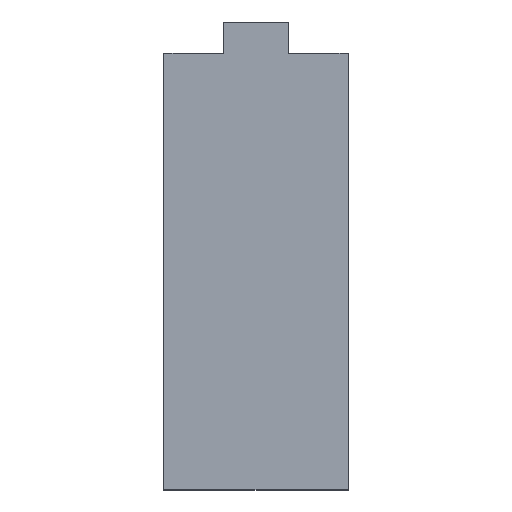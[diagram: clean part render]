
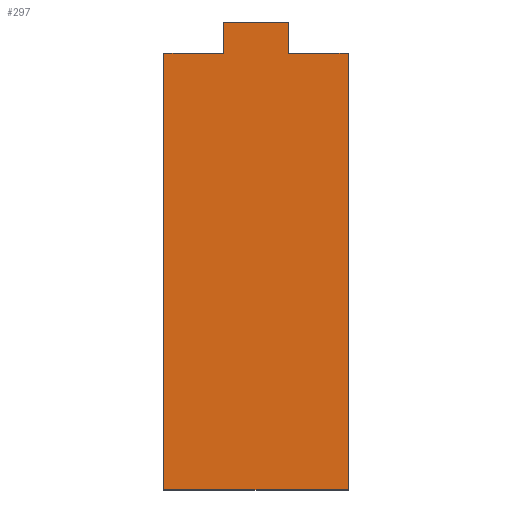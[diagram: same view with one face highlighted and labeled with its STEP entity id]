
A CAD part, top view. The second image highlights one B-rep face of the part: STEP entity #297.
In plain terms, the highlighted planar face has unit normal (0, 0, 1).
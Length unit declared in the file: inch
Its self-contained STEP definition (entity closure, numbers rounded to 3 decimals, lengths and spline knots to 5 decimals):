
#5 = DIRECTION ( 'NONE',  ( -1., 0., 0. ) ) ;
#11 = EDGE_CURVE ( 'NONE', #310, #309, #240, .T. ) ;
#15 = EDGE_CURVE ( 'NONE', #307, #330, #190, .T. ) ;
#16 = DIRECTION ( 'NONE',  ( 0., 1., 0. ) ) ;
#17 = CARTESIAN_POINT ( 'NONE',  ( 0.105, 1.4, 0.02 ) ) ;
#20 = CARTESIAN_POINT ( 'NONE',  ( 0., 0., 0.02 ) ) ;
#30 = CARTESIAN_POINT ( 'NONE',  ( -0.295, 1.4, 0.02 ) ) ;
#36 = PLANE ( 'NONE',  #134 ) ;
#39 = CARTESIAN_POINT ( 'NONE',  ( 0.295, 1.4, 0.02 ) ) ;
#58 = EDGE_CURVE ( 'NONE', #328, #325, #181, .T. ) ;
#60 = CARTESIAN_POINT ( 'NONE',  ( 0.295, 0., 0.02 ) ) ;
#61 = LINE ( 'NONE', #339, #225 ) ;
#72 = FACE_OUTER_BOUND ( 'NONE', #191, .T. ) ;
#79 = DIRECTION ( 'NONE',  ( 1., 0., 0. ) ) ;
#100 = CARTESIAN_POINT ( 'NONE',  ( 0.295, 0., 0.02 ) ) ;
#103 = EDGE_CURVE ( 'NONE', #322, #125, #168, .T. ) ;
#111 = VECTOR ( 'NONE', #228, 39.37008 ) ;
#118 = LINE ( 'NONE', #277, #111 ) ;
#125 = VERTEX_POINT ( 'NONE', #142 ) ;
#128 = DIRECTION ( 'NONE',  ( 1., 0., 0. ) ) ;
#131 = VECTOR ( 'NONE', #148, 39.37008 ) ;
#134 = AXIS2_PLACEMENT_3D ( 'NONE', #20, #283, #79 ) ;
#136 = VECTOR ( 'NONE', #5, 39.37008 ) ;
#142 = CARTESIAN_POINT ( 'NONE',  ( -0.105, 1.4, 0.02 ) ) ;
#143 = LINE ( 'NONE', #321, #136 ) ;
#147 = LINE ( 'NONE', #39, #131 ) ;
#148 = DIRECTION ( 'NONE',  ( -1., 0., 0. ) ) ;
#152 = EDGE_CURVE ( 'NONE', #125, #310, #143, .T. ) ;
#160 = VECTOR ( 'NONE', #271, 39.37008 ) ;
#162 = CARTESIAN_POINT ( 'NONE',  ( -0.105, 1.5, 0.02 ) ) ;
#168 = LINE ( 'NONE', #317, #160 ) ;
#174 = VECTOR ( 'NONE', #272, 39.37008 ) ;
#181 = LINE ( 'NONE', #17, #174 ) ;
#184 = VECTOR ( 'NONE', #16, 39.37008 ) ;
#189 = VECTOR ( 'NONE', #209, 39.37008 ) ;
#190 = LINE ( 'NONE', #100, #184 ) ;
#191 = EDGE_LOOP ( 'NONE', ( #275, #278, #281, #290, #291, #293, #299, #301 ) ) ;
#193 = EDGE_CURVE ( 'NONE', #330, #328, #147, .T. ) ;
#195 = CARTESIAN_POINT ( 'NONE',  ( 0.295, 1.4, 0.02 ) ) ;
#199 = CARTESIAN_POINT ( 'NONE',  ( 0.105, 1.4, 0.02 ) ) ;
#209 = DIRECTION ( 'NONE',  ( 0., -1., 0. ) ) ;
#225 = VECTOR ( 'NONE', #128, 39.37008 ) ;
#228 = DIRECTION ( 'NONE',  ( -1., 0., 0. ) ) ;
#240 = LINE ( 'NONE', #30, #189 ) ;
#254 = CARTESIAN_POINT ( 'NONE',  ( 0.105, 1.5, 0.02 ) ) ;
#262 = EDGE_CURVE ( 'NONE', #325, #322, #118, .T. ) ;
#271 = DIRECTION ( 'NONE',  ( 0., -1., 0. ) ) ;
#272 = DIRECTION ( 'NONE',  ( 0., 1., 0. ) ) ;
#275 = ORIENTED_EDGE ( 'NONE', *, *, #15, .T. ) ;
#277 = CARTESIAN_POINT ( 'NONE',  ( 0.105, 1.5, 0.02 ) ) ;
#278 = ORIENTED_EDGE ( 'NONE', *, *, #193, .T. ) ;
#281 = ORIENTED_EDGE ( 'NONE', *, *, #58, .T. ) ;
#283 = DIRECTION ( 'NONE',  ( 0., 0., 1. ) ) ;
#290 = ORIENTED_EDGE ( 'NONE', *, *, #262, .T. ) ;
#291 = ORIENTED_EDGE ( 'NONE', *, *, #103, .T. ) ;
#293 = ORIENTED_EDGE ( 'NONE', *, *, #152, .T. ) ;
#297 = ADVANCED_FACE ( 'NONE', ( #72 ), #36, .T. ) ;
#298 = CARTESIAN_POINT ( 'NONE',  ( -0.295, 0., 0.02 ) ) ;
#299 = ORIENTED_EDGE ( 'NONE', *, *, #11, .T. ) ;
#301 = ORIENTED_EDGE ( 'NONE', *, *, #314, .T. ) ;
#307 = VERTEX_POINT ( 'NONE', #60 ) ;
#309 = VERTEX_POINT ( 'NONE', #298 ) ;
#310 = VERTEX_POINT ( 'NONE', #336 ) ;
#314 = EDGE_CURVE ( 'NONE', #309, #307, #61, .T. ) ;
#317 = CARTESIAN_POINT ( 'NONE',  ( -0.105, 1.5, 0.02 ) ) ;
#321 = CARTESIAN_POINT ( 'NONE',  ( -0.105, 1.4, 0.02 ) ) ;
#322 = VERTEX_POINT ( 'NONE', #162 ) ;
#325 = VERTEX_POINT ( 'NONE', #254 ) ;
#328 = VERTEX_POINT ( 'NONE', #199 ) ;
#330 = VERTEX_POINT ( 'NONE', #195 ) ;
#336 = CARTESIAN_POINT ( 'NONE',  ( -0.295, 1.4, 0.02 ) ) ;
#339 = CARTESIAN_POINT ( 'NONE',  ( -0.295, 0., 0.02 ) ) ;
